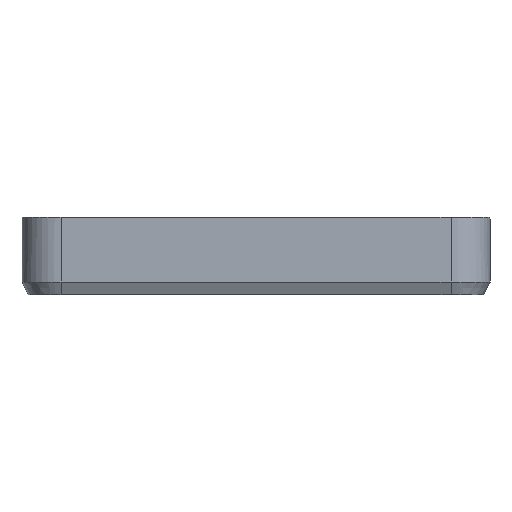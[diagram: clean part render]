
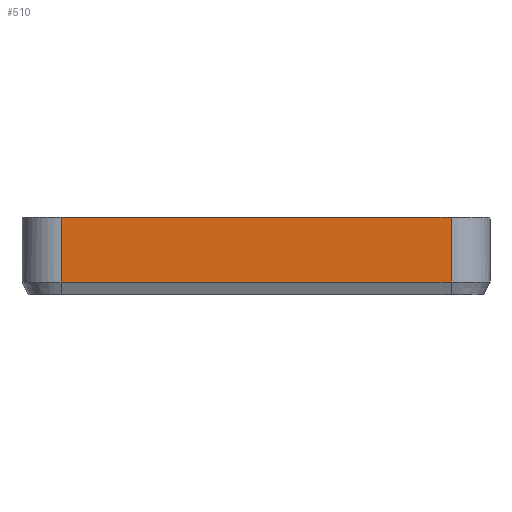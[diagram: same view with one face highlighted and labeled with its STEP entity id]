
A CAD part, left-side view. The second image highlights one B-rep face of the part: STEP entity #510.
In plain terms, the highlighted planar face has unit normal (-1, -0.001, 0).
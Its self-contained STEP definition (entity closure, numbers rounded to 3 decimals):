
#25=PLANE('',#576);
#59=FACE_OUTER_BOUND('',#89,.T.);
#89=EDGE_LOOP('',(#433,#434,#435,#436));
#104=LINE('',#774,#154);
#105=LINE('',#783,#155);
#120=LINE('',#834,#170);
#136=LINE('',#865,#186);
#154=VECTOR('',#615,10.);
#155=VECTOR('',#624,10.);
#170=VECTOR('',#673,10.);
#186=VECTOR('',#711,10.);
#235=VERTEX_POINT('',#771);
#236=VERTEX_POINT('',#773);
#239=VERTEX_POINT('',#780);
#240=VERTEX_POINT('',#782);
#280=EDGE_CURVE('',#235,#236,#104,.T.);
#284=EDGE_CURVE('',#239,#240,#105,.T.);
#311=EDGE_CURVE('',#240,#235,#120,.T.);
#327=EDGE_CURVE('',#239,#236,#136,.T.);
#433=ORIENTED_EDGE('',*,*,#311,.F.);
#434=ORIENTED_EDGE('',*,*,#284,.F.);
#435=ORIENTED_EDGE('',*,*,#327,.T.);
#436=ORIENTED_EDGE('',*,*,#280,.F.);
#510=ADVANCED_FACE('',(#59),#25,.F.);
#576=AXIS2_PLACEMENT_3D('',#864,#709,#710);
#615=DIRECTION('',(0.,0.,1.));
#624=DIRECTION('',(0.,0.,-1.));
#673=DIRECTION('',(-0.001,1.,0.));
#709=DIRECTION('center_axis',(1.,0.001,0.));
#710=DIRECTION('ref_axis',(0.,0.,-1.));
#711=DIRECTION('',(-0.001,1.,0.));
#771=CARTESIAN_POINT('',(40.728,46.593,1.));
#773=CARTESIAN_POINT('',(40.728,46.593,6.));
#774=CARTESIAN_POINT('',(40.728,46.593,11.807));
#780=CARTESIAN_POINT('',(40.747,16.593,6.));
#782=CARTESIAN_POINT('',(40.747,16.593,1.));
#783=CARTESIAN_POINT('',(40.747,16.593,11.807));
#834=CARTESIAN_POINT('',(40.747,16.592,1.));
#864=CARTESIAN_POINT('Origin',(40.756,1.593,7.));
#865=CARTESIAN_POINT('',(40.756,1.593,6.));
